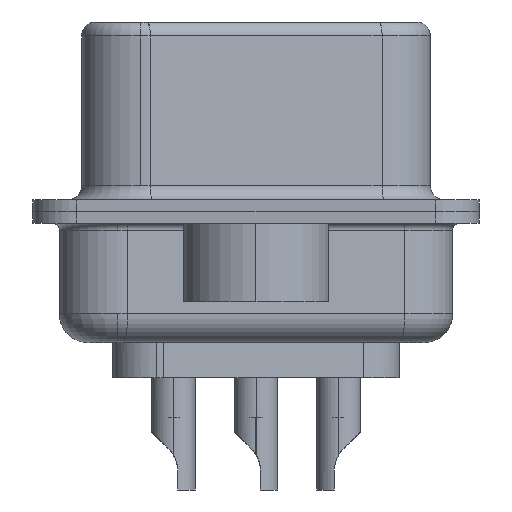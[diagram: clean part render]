
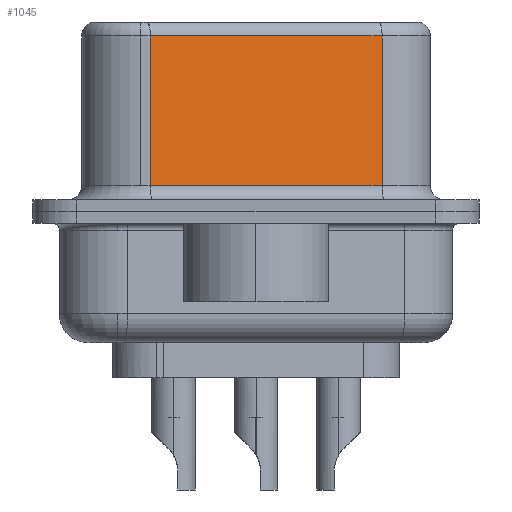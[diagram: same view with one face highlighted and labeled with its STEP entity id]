
A CAD part, left-side view. The second image highlights one B-rep face of the part: STEP entity #1045.
In plain terms, the highlighted planar face has unit normal (-0.985, -0.174, 0).
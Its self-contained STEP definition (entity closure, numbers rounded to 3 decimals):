
#460 = VERTEX_POINT ( 'NONE', #10206 ) ;
#573 = CARTESIAN_POINT ( 'NONE',  ( 3.73, 3.628, 6.02 ) ) ;
#1045 = ADVANCED_FACE ( 'NONE', ( #15822 ), #25073, .F. ) ;
#1817 = CARTESIAN_POINT ( 'NONE',  ( 5.132, -4.322, 0.9 ) ) ;
#2258 = EDGE_CURVE ( 'NONE', #6952, #27723, #23512, .T. ) ;
#3026 = EDGE_CURVE ( 'NONE', #460, #6952, #19815, .T. ) ;
#3180 = VECTOR ( 'NONE', #13362, 1000. ) ;
#3556 = DIRECTION ( 'NONE',  ( 0., 0., -1. ) ) ;
#4504 = VECTOR ( 'NONE', #3556, 1000. ) ;
#6289 = CARTESIAN_POINT ( 'NONE',  ( 3.73, 3.628, 0.9 ) ) ;
#6952 = VERTEX_POINT ( 'NONE', #573 ) ;
#7609 = LINE ( 'NONE', #25860, #4504 ) ;
#9869 = CARTESIAN_POINT ( 'NONE',  ( 3.73, 3.628, 6.52 ) ) ;
#10206 = CARTESIAN_POINT ( 'NONE',  ( 5.132, -4.322, 6.02 ) ) ;
#10871 = EDGE_CURVE ( 'NONE', #27723, #11016, #21849, .T. ) ;
#11016 = VERTEX_POINT ( 'NONE', #11076 ) ;
#11027 = DIRECTION ( 'NONE',  ( -0.174, 0.985, 0. ) ) ;
#11076 = CARTESIAN_POINT ( 'NONE',  ( 5.132, -4.322, 0.9 ) ) ;
#13098 = CARTESIAN_POINT ( 'NONE',  ( 5.132, -4.322, 6.52 ) ) ;
#13362 = DIRECTION ( 'NONE',  ( -0.174, 0.985, 0. ) ) ;
#15175 = AXIS2_PLACEMENT_3D ( 'NONE', #13098, #22406, #11027 ) ;
#15822 = FACE_OUTER_BOUND ( 'NONE', #19253, .T. ) ;
#16405 = EDGE_CURVE ( 'NONE', #460, #11016, #7609, .T. ) ;
#19253 = EDGE_LOOP ( 'NONE', ( #23543, #24955, #28472, #20199 ) ) ;
#19758 = DIRECTION ( 'NONE',  ( 0.174, -0.985, 0. ) ) ;
#19815 = LINE ( 'NONE', #24453, #3180 ) ;
#20199 = ORIENTED_EDGE ( 'NONE', *, *, #10871, .T. ) ;
#21849 = LINE ( 'NONE', #1817, #26161 ) ;
#22406 = DIRECTION ( 'NONE',  ( 0.985, 0.174, 0. ) ) ;
#23286 = VECTOR ( 'NONE', #27972, 1000. ) ;
#23512 = LINE ( 'NONE', #9869, #23286 ) ;
#23543 = ORIENTED_EDGE ( 'NONE', *, *, #16405, .F. ) ;
#24453 = CARTESIAN_POINT ( 'NONE',  ( 5.132, -4.322, 6.02 ) ) ;
#24955 = ORIENTED_EDGE ( 'NONE', *, *, #3026, .T. ) ;
#25073 = PLANE ( 'NONE',  #15175 ) ;
#25860 = CARTESIAN_POINT ( 'NONE',  ( 5.132, -4.322, 6.52 ) ) ;
#26161 = VECTOR ( 'NONE', #19758, 1000. ) ;
#27723 = VERTEX_POINT ( 'NONE', #6289 ) ;
#27972 = DIRECTION ( 'NONE',  ( 0., 0., -1. ) ) ;
#28472 = ORIENTED_EDGE ( 'NONE', *, *, #2258, .T. ) ;
